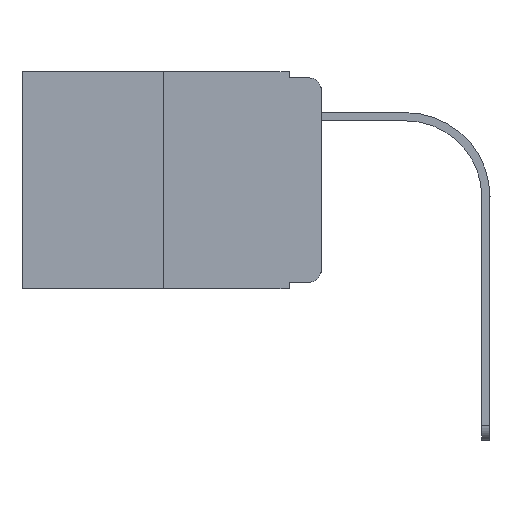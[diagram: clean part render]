
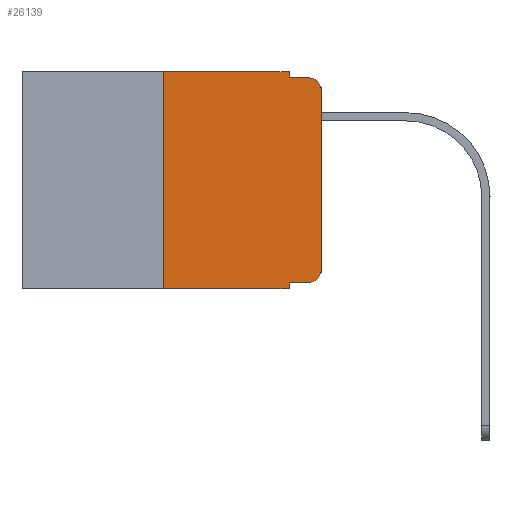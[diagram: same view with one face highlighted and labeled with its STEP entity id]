
A CAD part, left-side view. The second image highlights one B-rep face of the part: STEP entity #26139.
In plain terms, the highlighted planar face has unit normal (-1, 0, 0).
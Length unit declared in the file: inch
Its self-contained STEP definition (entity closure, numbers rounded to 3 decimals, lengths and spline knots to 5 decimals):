
#1237 = CARTESIAN_POINT ( 'NONE',  ( 0., 0.051, 0. ) ) ;
#1646 = CARTESIAN_POINT ( 'NONE',  ( 0., 0., 0. ) ) ;
#1648 = LINE ( 'NONE', #7749, #4268 ) ;
#1943 = VECTOR ( 'NONE', #16931, 39.37008 ) ;
#2089 = VERTEX_POINT ( 'NONE', #1237 ) ;
#2428 = CARTESIAN_POINT ( 'NONE',  ( 0., 0.25, 0. ) ) ;
#2474 = VERTEX_POINT ( 'NONE', #11441 ) ;
#3028 = DIRECTION ( 'NONE',  ( -1., 0., 0. ) ) ;
#4268 = VECTOR ( 'NONE', #25994, 39.37008 ) ;
#4469 = VECTOR ( 'NONE', #12290, 39.37008 ) ;
#4529 = AXIS2_PLACEMENT_3D ( 'NONE', #21462, #4850, #19599 ) ;
#4619 = LINE ( 'NONE', #24979, #24049 ) ;
#4850 = DIRECTION ( 'NONE',  ( 1., 0., 0. ) ) ;
#5398 = EDGE_CURVE ( 'NONE', #18255, #13277, #7779, .T. ) ;
#5884 = EDGE_CURVE ( 'NONE', #8836, #6069, #1648, .T. ) ;
#6069 = VERTEX_POINT ( 'NONE', #11187 ) ;
#6827 = CARTESIAN_POINT ( 'NONE',  ( 0., 0.473, -0.343 ) ) ;
#7153 = CARTESIAN_POINT ( 'NONE',  ( 0., 0.02, -0.03 ) ) ;
#7214 = ORIENTED_EDGE ( 'NONE', *, *, #18693, .T. ) ;
#7303 = ORIENTED_EDGE ( 'NONE', *, *, #5398, .F. ) ;
#7395 = ORIENTED_EDGE ( 'NONE', *, *, #19660, .F. ) ;
#7427 = EDGE_LOOP ( 'NONE', ( #14070, #7432, #7303, #21464, #23264, #7395, #10850, #11146, #10555, #7214 ) ) ;
#7432 = ORIENTED_EDGE ( 'NONE', *, *, #20025, .T. ) ;
#7610 = VERTEX_POINT ( 'NONE', #13457 ) ;
#7749 = CARTESIAN_POINT ( 'NONE',  ( 0., 0.051, 0. ) ) ;
#7779 = LINE ( 'NONE', #19639, #26153 ) ;
#8836 = VERTEX_POINT ( 'NONE', #15351 ) ;
#9885 = LINE ( 'NONE', #1646, #13341 ) ;
#10017 = AXIS2_PLACEMENT_3D ( 'NONE', #12590, #18987, #20735 ) ;
#10239 = EDGE_CURVE ( 'NONE', #7610, #2474, #9885, .T. ) ;
#10555 = ORIENTED_EDGE ( 'NONE', *, *, #24704, .T. ) ;
#10850 = ORIENTED_EDGE ( 'NONE', *, *, #16080, .T. ) ;
#11146 = ORIENTED_EDGE ( 'NONE', *, *, #5884, .F. ) ;
#11155 = CARTESIAN_POINT ( 'NONE',  ( 0., 0.25, 0. ) ) ;
#11187 = CARTESIAN_POINT ( 'NONE',  ( 0., 0.051, -0.343 ) ) ;
#11425 = LINE ( 'NONE', #11155, #18056 ) ;
#11441 = CARTESIAN_POINT ( 'NONE',  ( 0., 0., -0.03 ) ) ;
#12290 = DIRECTION ( 'NONE',  ( 0., -1., 0. ) ) ;
#12543 = CIRCLE ( 'NONE', #10017, 0.02 ) ;
#12590 = CARTESIAN_POINT ( 'NONE',  ( 0., 0.02, -0.313 ) ) ;
#12775 = CARTESIAN_POINT ( 'NONE',  ( 0., 0.473, 0. ) ) ;
#12872 = CARTESIAN_POINT ( 'NONE',  ( 0., 0.051, -0.01 ) ) ;
#12937 = VERTEX_POINT ( 'NONE', #14133 ) ;
#12985 = VERTEX_POINT ( 'NONE', #2428 ) ;
#13186 = LINE ( 'NONE', #12775, #1943 ) ;
#13277 = VERTEX_POINT ( 'NONE', #23940 ) ;
#13341 = VECTOR ( 'NONE', #18273, 39.37008 ) ;
#13457 = CARTESIAN_POINT ( 'NONE',  ( 0., 0., -0.313 ) ) ;
#13821 = CIRCLE ( 'NONE', #21913, 0.02 ) ;
#14070 = ORIENTED_EDGE ( 'NONE', *, *, #10239, .T. ) ;
#14133 = CARTESIAN_POINT ( 'NONE',  ( 0., 0.02, -0.333 ) ) ;
#15351 = CARTESIAN_POINT ( 'NONE',  ( 0., 0.051, -0.333 ) ) ;
#15907 = DIRECTION ( 'NONE',  ( 0., -1., 0. ) ) ;
#16080 = EDGE_CURVE ( 'NONE', #22421, #6069, #20943, .T. ) ;
#16332 = DIRECTION ( 'NONE',  ( 0., 0., -1. ) ) ;
#16532 = VECTOR ( 'NONE', #23205, 39.37008 ) ;
#16931 = DIRECTION ( 'NONE',  ( 0., -1., 0. ) ) ;
#18056 = VECTOR ( 'NONE', #21557, 39.37008 ) ;
#18255 = VERTEX_POINT ( 'NONE', #12872 ) ;
#18273 = DIRECTION ( 'NONE',  ( 0., 0., 1. ) ) ;
#18659 = EDGE_CURVE ( 'NONE', #2089, #18255, #4619, .T. ) ;
#18693 = EDGE_CURVE ( 'NONE', #12937, #7610, #12543, .T. ) ;
#18927 = CARTESIAN_POINT ( 'NONE',  ( 0., 0.051, -0.333 ) ) ;
#18987 = DIRECTION ( 'NONE',  ( -1., 0., 0. ) ) ;
#19468 = PLANE ( 'NONE',  #4529 ) ;
#19599 = DIRECTION ( 'NONE',  ( 0., 0., -1. ) ) ;
#19639 = CARTESIAN_POINT ( 'NONE',  ( 0., 0.051, -0.01 ) ) ;
#19660 = EDGE_CURVE ( 'NONE', #22421, #12985, #11425, .T. ) ;
#20025 = EDGE_CURVE ( 'NONE', #2474, #13277, #13821, .T. ) ;
#20211 = EDGE_CURVE ( 'NONE', #12985, #2089, #13186, .T. ) ;
#20417 = LINE ( 'NONE', #18927, #4469 ) ;
#20735 = DIRECTION ( 'NONE',  ( 0., 0., -1. ) ) ;
#20943 = LINE ( 'NONE', #6827, #16532 ) ;
#21462 = CARTESIAN_POINT ( 'NONE',  ( 0., 0.473, 0. ) ) ;
#21464 = ORIENTED_EDGE ( 'NONE', *, *, #18659, .F. ) ;
#21557 = DIRECTION ( 'NONE',  ( 0., 0., 1. ) ) ;
#21913 = AXIS2_PLACEMENT_3D ( 'NONE', #7153, #3028, #23396 ) ;
#22421 = VERTEX_POINT ( 'NONE', #25773 ) ;
#23089 = FACE_OUTER_BOUND ( 'NONE', #7427, .T. ) ;
#23205 = DIRECTION ( 'NONE',  ( 0., -1., 0. ) ) ;
#23264 = ORIENTED_EDGE ( 'NONE', *, *, #20211, .F. ) ;
#23396 = DIRECTION ( 'NONE',  ( 0., 0., -1. ) ) ;
#23940 = CARTESIAN_POINT ( 'NONE',  ( 0., 0.02, -0.01 ) ) ;
#24049 = VECTOR ( 'NONE', #16332, 39.37008 ) ;
#24704 = EDGE_CURVE ( 'NONE', #8836, #12937, #20417, .T. ) ;
#24979 = CARTESIAN_POINT ( 'NONE',  ( 0., 0.051, 0. ) ) ;
#25773 = CARTESIAN_POINT ( 'NONE',  ( 0., 0.25, -0.343 ) ) ;
#25994 = DIRECTION ( 'NONE',  ( 0., 0., -1. ) ) ;
#26139 = ADVANCED_FACE ( 'NONE', ( #23089 ), #19468, .F. ) ;
#26153 = VECTOR ( 'NONE', #15907, 39.37008 ) ;
